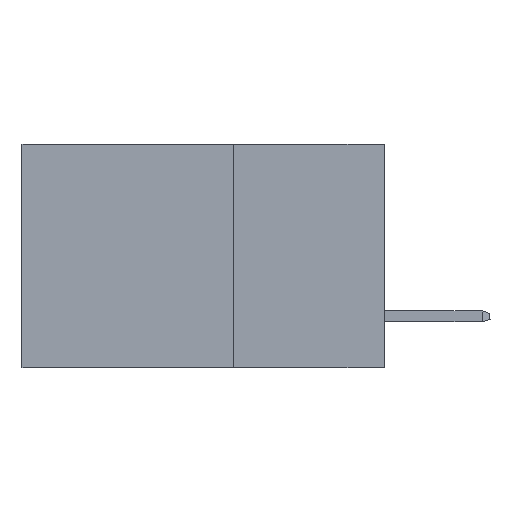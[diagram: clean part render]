
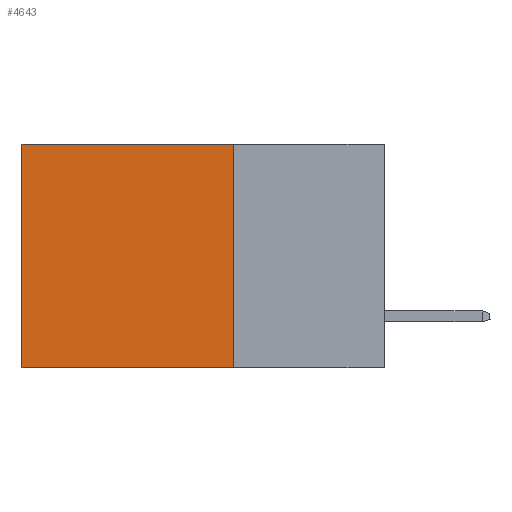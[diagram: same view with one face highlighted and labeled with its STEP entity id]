
A CAD part, left-side view. The second image highlights one B-rep face of the part: STEP entity #4643.
In plain terms, the highlighted planar face has unit normal (-1, 0, 0).
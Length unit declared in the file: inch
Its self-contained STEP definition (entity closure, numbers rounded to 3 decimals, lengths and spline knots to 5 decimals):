
#447 = VECTOR ( 'NONE', #4631, 39.37008 ) ;
#3287 = LINE ( 'NONE', #29495, #6693 ) ;
#3526 = CARTESIAN_POINT ( 'NONE',  ( 0.298, 0.6, 0. ) ) ;
#4127 = DIRECTION ( 'NONE',  ( 0., 0., -1. ) ) ;
#4323 = CARTESIAN_POINT ( 'NONE',  ( 0.298, 0.25, -0.37 ) ) ;
#4631 = DIRECTION ( 'NONE',  ( 0., 1., 0. ) ) ;
#4643 = ADVANCED_FACE ( 'NONE', ( #7031 ), #23277, .F. ) ;
#5030 = CARTESIAN_POINT ( 'NONE',  ( 0.298, 0.6, -0.37 ) ) ;
#6299 = EDGE_CURVE ( 'NONE', #9116, #14745, #30250, .T. ) ;
#6693 = VECTOR ( 'NONE', #17508, 39.37008 ) ;
#7031 = FACE_OUTER_BOUND ( 'NONE', #28146, .T. ) ;
#7803 = VECTOR ( 'NONE', #11450, 39.37008 ) ;
#8217 = EDGE_CURVE ( 'NONE', #14137, #14745, #3287, .T. ) ;
#9116 = VERTEX_POINT ( 'NONE', #19211 ) ;
#9154 = DIRECTION ( 'NONE',  ( 0., 1., 0. ) ) ;
#10576 = CARTESIAN_POINT ( 'NONE',  ( 0.298, 0.25, 0. ) ) ;
#10748 = ORIENTED_EDGE ( 'NONE', *, *, #16123, .T. ) ;
#11219 = CARTESIAN_POINT ( 'NONE',  ( 0.298, 0.25, 0. ) ) ;
#11450 = DIRECTION ( 'NONE',  ( 0., 0., -1. ) ) ;
#14047 = LINE ( 'NONE', #21234, #30220 ) ;
#14137 = VERTEX_POINT ( 'NONE', #3526 ) ;
#14203 = AXIS2_PLACEMENT_3D ( 'NONE', #11219, #18331, #4127 ) ;
#14745 = VERTEX_POINT ( 'NONE', #5030 ) ;
#15841 = CARTESIAN_POINT ( 'NONE',  ( 0.298, 0.25, 0. ) ) ;
#16123 = EDGE_CURVE ( 'NONE', #23385, #14137, #14047, .T. ) ;
#17508 = DIRECTION ( 'NONE',  ( 0., 0., -1. ) ) ;
#18331 = DIRECTION ( 'NONE',  ( 1., 0., 0. ) ) ;
#19211 = CARTESIAN_POINT ( 'NONE',  ( 0.298, 0.25, -0.37 ) ) ;
#19515 = LINE ( 'NONE', #15841, #7803 ) ;
#21234 = CARTESIAN_POINT ( 'NONE',  ( 0.298, 0.25, 0. ) ) ;
#21672 = ORIENTED_EDGE ( 'NONE', *, *, #6299, .F. ) ;
#22520 = ORIENTED_EDGE ( 'NONE', *, *, #22983, .F. ) ;
#22983 = EDGE_CURVE ( 'NONE', #23385, #9116, #19515, .T. ) ;
#23277 = PLANE ( 'NONE',  #14203 ) ;
#23385 = VERTEX_POINT ( 'NONE', #10576 ) ;
#27659 = ORIENTED_EDGE ( 'NONE', *, *, #8217, .T. ) ;
#28146 = EDGE_LOOP ( 'NONE', ( #27659, #21672, #22520, #10748 ) ) ;
#29495 = CARTESIAN_POINT ( 'NONE',  ( 0.298, 0.6, 0. ) ) ;
#30220 = VECTOR ( 'NONE', #9154, 39.37008 ) ;
#30250 = LINE ( 'NONE', #4323, #447 ) ;
